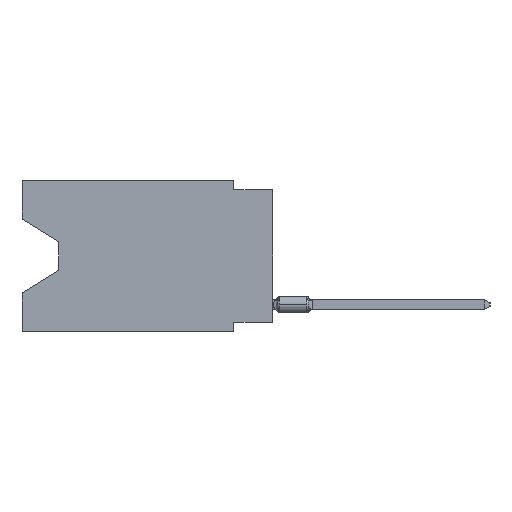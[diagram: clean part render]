
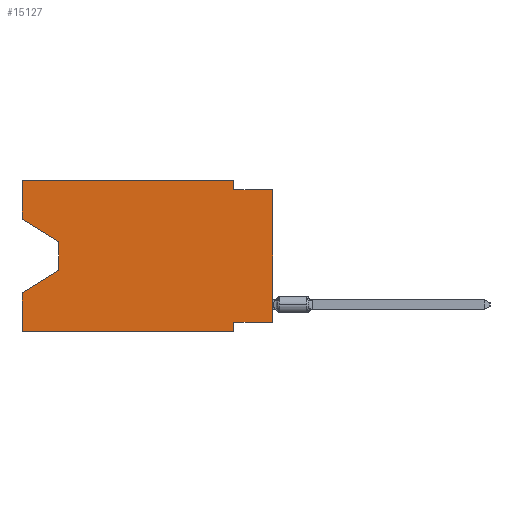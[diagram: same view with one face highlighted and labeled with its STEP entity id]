
A CAD part, left-side view. The second image highlights one B-rep face of the part: STEP entity #15127.
In plain terms, the highlighted planar face has unit normal (-1, 0, 0).
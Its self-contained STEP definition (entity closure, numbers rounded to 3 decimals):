
#352 = EDGE_CURVE ( 'NONE', #34729, #6006, #42347, .T. ) ;
#1217 = LINE ( 'NONE', #27582, #23129 ) ;
#1481 = EDGE_CURVE ( 'NONE', #28489, #62516, #41524, .T. ) ;
#2222 = DIRECTION ( 'NONE',  ( 0., 0., 1. ) ) ;
#2815 = DIRECTION ( 'NONE',  ( 1., 0., 0. ) ) ;
#5347 = EDGE_CURVE ( 'NONE', #83439, #57519, #45550, .T. ) ;
#6006 = VERTEX_POINT ( 'NONE', #26090 ) ;
#6252 = CARTESIAN_POINT ( 'NONE',  ( 0., 16.383, -9.906 ) ) ;
#9291 = CARTESIAN_POINT ( 'NONE',  ( 0., 0., -0.635 ) ) ;
#10137 = PLANE ( 'NONE',  #28148 ) ;
#12083 = VECTOR ( 'NONE', #81367, 1000. ) ;
#13464 = EDGE_CURVE ( 'NONE', #73426, #57519, #41048, .T. ) ;
#14173 = ORIENTED_EDGE ( 'NONE', *, *, #48849, .T. ) ;
#14556 = DIRECTION ( 'NONE',  ( 0., 0.855, -0.519 ) ) ;
#15081 = CARTESIAN_POINT ( 'NONE',  ( 0., 16.383, -7.36 ) ) ;
#15127 = ADVANCED_FACE ( 'NONE', ( #21402 ), #10137, .F. ) ;
#15538 = ORIENTED_EDGE ( 'NONE', *, *, #352, .F. ) ;
#16008 = CARTESIAN_POINT ( 'NONE',  ( 0., 13.97, -4.013 ) ) ;
#16060 = VECTOR ( 'NONE', #31919, 1000. ) ;
#17764 = VECTOR ( 'NONE', #51617, 1000. ) ;
#18290 = ORIENTED_EDGE ( 'NONE', *, *, #46901, .F. ) ;
#19708 = EDGE_CURVE ( 'NONE', #6006, #51828, #53367, .T. ) ;
#20678 = EDGE_CURVE ( 'NONE', #28489, #73426, #1217, .T. ) ;
#21402 = FACE_OUTER_BOUND ( 'NONE', #60199, .T. ) ;
#22097 = LINE ( 'NONE', #16008, #63094 ) ;
#22122 = CARTESIAN_POINT ( 'NONE',  ( 0., 13.97, -5.893 ) ) ;
#23129 = VECTOR ( 'NONE', #32764, 1000. ) ;
#24613 = LINE ( 'NONE', #85021, #16060 ) ;
#26090 = CARTESIAN_POINT ( 'NONE',  ( 0., 16.383, 0. ) ) ;
#26449 = ORIENTED_EDGE ( 'NONE', *, *, #5347, .T. ) ;
#26573 = LINE ( 'NONE', #52895, #17764 ) ;
#27582 = CARTESIAN_POINT ( 'NONE',  ( 0., 0., -9.271 ) ) ;
#28148 = AXIS2_PLACEMENT_3D ( 'NONE', #35634, #2815, #36464 ) ;
#28489 = VERTEX_POINT ( 'NONE', #54966 ) ;
#28690 = LINE ( 'NONE', #34735, #12083 ) ;
#29836 = ORIENTED_EDGE ( 'NONE', *, *, #46684, .F. ) ;
#30240 = DIRECTION ( 'NONE',  ( 0., 0., 1. ) ) ;
#30661 = CARTESIAN_POINT ( 'NONE',  ( 0., 16.383, 0. ) ) ;
#31919 = DIRECTION ( 'NONE',  ( 0., 0., -1. ) ) ;
#32764 = DIRECTION ( 'NONE',  ( 0., 1., 0. ) ) ;
#34147 = DIRECTION ( 'NONE',  ( 0., 0., -1. ) ) ;
#34729 = VERTEX_POINT ( 'NONE', #61615 ) ;
#34735 = CARTESIAN_POINT ( 'NONE',  ( 0., 16.383, 0. ) ) ;
#34850 = LINE ( 'NONE', #81069, #64002 ) ;
#34968 = CARTESIAN_POINT ( 'NONE',  ( 0., 2.54, -9.906 ) ) ;
#35634 = CARTESIAN_POINT ( 'NONE',  ( 0., 16.383, 0. ) ) ;
#36464 = DIRECTION ( 'NONE',  ( 0., 0., -1. ) ) ;
#39546 = DIRECTION ( 'NONE',  ( 0., -1., 0. ) ) ;
#40710 = CARTESIAN_POINT ( 'NONE',  ( 0., 2.54, -0.635 ) ) ;
#40753 = ORIENTED_EDGE ( 'NONE', *, *, #13464, .F. ) ;
#41048 = LINE ( 'NONE', #68227, #66524 ) ;
#41524 = LINE ( 'NONE', #61380, #63426 ) ;
#42347 = LINE ( 'NONE', #30661, #44002 ) ;
#42907 = EDGE_CURVE ( 'NONE', #83439, #55443, #28690, .T. ) ;
#43261 = VERTEX_POINT ( 'NONE', #22122 ) ;
#44002 = VECTOR ( 'NONE', #30240, 1000. ) ;
#44287 = EDGE_CURVE ( 'NONE', #34729, #58070, #26573, .T. ) ;
#44942 = EDGE_CURVE ( 'NONE', #43261, #55443, #34850, .T. ) ;
#45497 = CARTESIAN_POINT ( 'NONE',  ( 0., 2.54, -9.271 ) ) ;
#45550 = LINE ( 'NONE', #6252, #57027 ) ;
#46684 = EDGE_CURVE ( 'NONE', #63908, #62516, #69038, .T. ) ;
#46901 = EDGE_CURVE ( 'NONE', #51828, #63908, #24613, .T. ) ;
#48849 = EDGE_CURVE ( 'NONE', #58070, #43261, #22097, .T. ) ;
#49137 = ORIENTED_EDGE ( 'NONE', *, *, #44287, .T. ) ;
#50493 = VECTOR ( 'NONE', #39546, 1000. ) ;
#50667 = ORIENTED_EDGE ( 'NONE', *, *, #20678, .F. ) ;
#51617 = DIRECTION ( 'NONE',  ( 0., -0.855, -0.519 ) ) ;
#51665 = ORIENTED_EDGE ( 'NONE', *, *, #1481, .T. ) ;
#51753 = ORIENTED_EDGE ( 'NONE', *, *, #44942, .T. ) ;
#51828 = VERTEX_POINT ( 'NONE', #59446 ) ;
#52516 = CARTESIAN_POINT ( 'NONE',  ( 0., 16.383, 0. ) ) ;
#52895 = CARTESIAN_POINT ( 'NONE',  ( 0., 16.383, -2.546 ) ) ;
#53367 = LINE ( 'NONE', #52516, #50493 ) ;
#54966 = CARTESIAN_POINT ( 'NONE',  ( 0., 0., -9.271 ) ) ;
#55443 = VERTEX_POINT ( 'NONE', #15081 ) ;
#57027 = VECTOR ( 'NONE', #71892, 1000. ) ;
#57354 = VECTOR ( 'NONE', #69446, 1000. ) ;
#57519 = VERTEX_POINT ( 'NONE', #34968 ) ;
#58070 = VERTEX_POINT ( 'NONE', #78416 ) ;
#59446 = CARTESIAN_POINT ( 'NONE',  ( 0., 2.54, 0. ) ) ;
#60199 = EDGE_LOOP ( 'NONE', ( #49137, #14173, #51753, #82166, #26449, #40753, #50667, #51665, #29836, #18290, #62851, #15538 ) ) ;
#61380 = CARTESIAN_POINT ( 'NONE',  ( 0., 0., 0. ) ) ;
#61615 = CARTESIAN_POINT ( 'NONE',  ( 0., 16.383, -2.546 ) ) ;
#62516 = VERTEX_POINT ( 'NONE', #9291 ) ;
#62851 = ORIENTED_EDGE ( 'NONE', *, *, #19708, .F. ) ;
#63094 = VECTOR ( 'NONE', #74349, 1000. ) ;
#63426 = VECTOR ( 'NONE', #2222, 1000. ) ;
#63572 = CARTESIAN_POINT ( 'NONE',  ( 0., 16.383, -9.906 ) ) ;
#63908 = VERTEX_POINT ( 'NONE', #40710 ) ;
#64002 = VECTOR ( 'NONE', #14556, 1000. ) ;
#66524 = VECTOR ( 'NONE', #34147, 1000. ) ;
#68227 = CARTESIAN_POINT ( 'NONE',  ( 0., 2.54, -9.906 ) ) ;
#69038 = LINE ( 'NONE', #82419, #57354 ) ;
#69446 = DIRECTION ( 'NONE',  ( 0., -1., 0. ) ) ;
#71892 = DIRECTION ( 'NONE',  ( 0., -1., 0. ) ) ;
#73426 = VERTEX_POINT ( 'NONE', #45497 ) ;
#74349 = DIRECTION ( 'NONE',  ( 0., 0., -1. ) ) ;
#78416 = CARTESIAN_POINT ( 'NONE',  ( 0., 13.97, -4.013 ) ) ;
#81069 = CARTESIAN_POINT ( 'NONE',  ( 0., 13.97, -5.893 ) ) ;
#81367 = DIRECTION ( 'NONE',  ( 0., 0., 1. ) ) ;
#82166 = ORIENTED_EDGE ( 'NONE', *, *, #42907, .F. ) ;
#82419 = CARTESIAN_POINT ( 'NONE',  ( 0., 0., -0.635 ) ) ;
#83439 = VERTEX_POINT ( 'NONE', #63572 ) ;
#85021 = CARTESIAN_POINT ( 'NONE',  ( 0., 2.54, 0. ) ) ;
